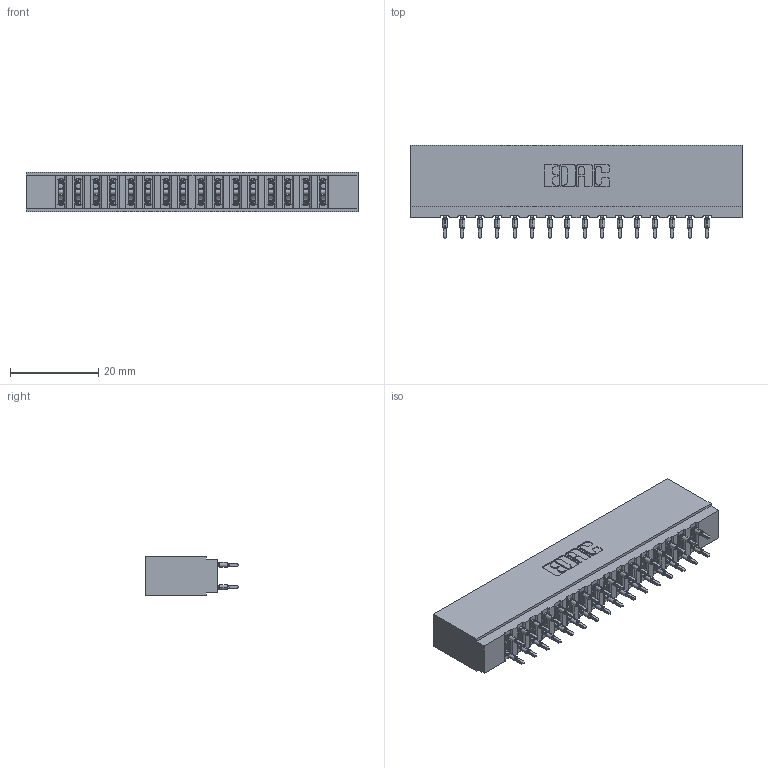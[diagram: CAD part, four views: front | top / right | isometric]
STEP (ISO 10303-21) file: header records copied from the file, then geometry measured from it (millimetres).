
FILE_DESCRIPTION (( 'STEP AP203' ), '1' );
FILE_NAME ('737-032-560-201.STEP', '2020-09-11T00:19:17', ( '' ), ( '' ), 'SwSTEP 2.0', 'SolidWorks 2020', '' );
FILE_SCHEMA (( 'CONFIG_CONTROL_DESIGN' ));
Length unit declared in the file: inch
Products named in the file (3): 737 Part_Insulator Option - 01; 737-032-560-201; 745-292-001_560
Assembly tree (33 placements, depth 2):
  737-032-560-201
    737 Part_Insulator Option - 01
    745-292-001_560  x32
Bounding box: 75.23 x 21.22 x 8.89 mm (x, y, z)
Volume: 7719.8 mm3; surface area: 11209.2 mm2
Topology: 33 solids, 33 shells, 3262 faces, 8927 edges, 5674 vertices
Faces by surface type: plane 1702, cylinder 728, bspline 640, torus 192
Entity records: 31310 total; most frequent: CARTESIAN_POINT 5947, ORIENTED_EDGE 5330, DIRECTION 4679, EDGE_CURVE 2665, VECTOR 2379, LINE 2379, VERTEX_POINT 1706, AXIS2_PLACEMENT_3D 1150
